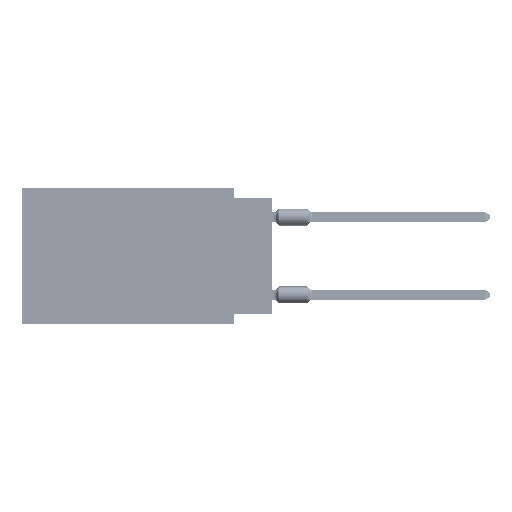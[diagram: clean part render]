
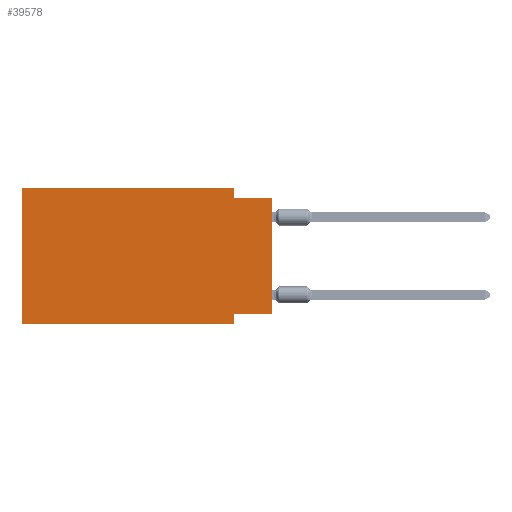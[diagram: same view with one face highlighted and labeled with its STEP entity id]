
A CAD part, left-side view. The second image highlights one B-rep face of the part: STEP entity #39578.
In plain terms, the highlighted planar face has unit normal (-1, 0, 0).
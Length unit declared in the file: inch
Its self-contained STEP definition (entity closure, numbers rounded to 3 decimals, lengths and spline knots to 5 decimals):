
#1362 = VERTEX_POINT ( 'NONE', #86195 ) ;
#1714 = DIRECTION ( 'NONE',  ( 0., -1., 0. ) ) ;
#3912 = EDGE_CURVE ( 'NONE', #1362, #72375, #49674, .T. ) ;
#4605 = CARTESIAN_POINT ( 'NONE',  ( 0., 0.1, 0. ) ) ;
#5267 = CARTESIAN_POINT ( 'NONE',  ( 0., 0., -0.025 ) ) ;
#7550 = CARTESIAN_POINT ( 'NONE',  ( 0., 0.645, 0. ) ) ;
#8729 = CARTESIAN_POINT ( 'NONE',  ( 0., 0.645, 0. ) ) ;
#9142 = LINE ( 'NONE', #7550, #26020 ) ;
#12862 = CARTESIAN_POINT ( 'NONE',  ( 0., 0.645, 0. ) ) ;
#16244 = DIRECTION ( 'NONE',  ( 0., 0., 1. ) ) ;
#19737 = CARTESIAN_POINT ( 'NONE',  ( 0., 0.1, -0.35 ) ) ;
#21460 = EDGE_CURVE ( 'NONE', #58977, #82890, #29327, .T. ) ;
#22205 = VERTEX_POINT ( 'NONE', #104727 ) ;
#22870 = LINE ( 'NONE', #71292, #58501 ) ;
#23210 = ORIENTED_EDGE ( 'NONE', *, *, #62067, .T. ) ;
#23271 = VERTEX_POINT ( 'NONE', #83440 ) ;
#23874 = CARTESIAN_POINT ( 'NONE',  ( 0., 0.1, -0.025 ) ) ;
#24362 = CARTESIAN_POINT ( 'NONE',  ( 0., 0.645, 0. ) ) ;
#26020 = VECTOR ( 'NONE', #67216, 39.37008 ) ;
#29327 = LINE ( 'NONE', #4605, #31275 ) ;
#29997 = VERTEX_POINT ( 'NONE', #53383 ) ;
#31275 = VECTOR ( 'NONE', #70201, 39.37008 ) ;
#31969 = VERTEX_POINT ( 'NONE', #24362 ) ;
#35643 = CARTESIAN_POINT ( 'NONE',  ( 0., 0.1, -0.35 ) ) ;
#38148 = DIRECTION ( 'NONE',  ( 0., 0., -1. ) ) ;
#39578 = ADVANCED_FACE ( 'NONE', ( #69886 ), #61796, .F. ) ;
#42580 = LINE ( 'NONE', #5267, #50592 ) ;
#45679 = DIRECTION ( 'NONE',  ( 1., 0., 0. ) ) ;
#49674 = LINE ( 'NONE', #35643, #68982 ) ;
#50445 = VECTOR ( 'NONE', #51310, 39.37008 ) ;
#50592 = VECTOR ( 'NONE', #1714, 39.37008 ) ;
#51310 = DIRECTION ( 'NONE',  ( 0., -1., 0. ) ) ;
#53383 = CARTESIAN_POINT ( 'NONE',  ( 0., 0., -0.325 ) ) ;
#57918 = CARTESIAN_POINT ( 'NONE',  ( 0., 0., -0.325 ) ) ;
#58501 = VECTOR ( 'NONE', #64800, 39.37008 ) ;
#58977 = VERTEX_POINT ( 'NONE', #88517 ) ;
#59296 = DIRECTION ( 'NONE',  ( 0., 0., -1. ) ) ;
#61796 = PLANE ( 'NONE',  #67469 ) ;
#62067 = EDGE_CURVE ( 'NONE', #23271, #72375, #84107, .T. ) ;
#64331 = EDGE_CURVE ( 'NONE', #82890, #22205, #42580, .T. ) ;
#64800 = DIRECTION ( 'NONE',  ( 0., 0., 1. ) ) ;
#66525 = DIRECTION ( 'NONE',  ( 0., 1., 0. ) ) ;
#66859 = VECTOR ( 'NONE', #16244, 39.37008 ) ;
#67216 = DIRECTION ( 'NONE',  ( 0., -1., 0. ) ) ;
#67469 = AXIS2_PLACEMENT_3D ( 'NONE', #12862, #45679, #38148 ) ;
#68235 = ORIENTED_EDGE ( 'NONE', *, *, #104474, .F. ) ;
#68982 = VECTOR ( 'NONE', #59296, 39.37008 ) ;
#69886 = FACE_OUTER_BOUND ( 'NONE', #101928, .T. ) ;
#70201 = DIRECTION ( 'NONE',  ( 0., 0., -1. ) ) ;
#70419 = VECTOR ( 'NONE', #66525, 39.37008 ) ;
#70621 = ORIENTED_EDGE ( 'NONE', *, *, #21460, .F. ) ;
#71292 = CARTESIAN_POINT ( 'NONE',  ( 0., 0., 0. ) ) ;
#72375 = VERTEX_POINT ( 'NONE', #19737 ) ;
#73145 = ORIENTED_EDGE ( 'NONE', *, *, #105015, .F. ) ;
#74070 = LINE ( 'NONE', #57918, #70419 ) ;
#74323 = LINE ( 'NONE', #8729, #66859 ) ;
#77754 = ORIENTED_EDGE ( 'NONE', *, *, #105225, .T. ) ;
#78158 = CARTESIAN_POINT ( 'NONE',  ( 0., 0.645, -0.35 ) ) ;
#82890 = VERTEX_POINT ( 'NONE', #23874 ) ;
#83440 = CARTESIAN_POINT ( 'NONE',  ( 0., 0.645, -0.35 ) ) ;
#84107 = LINE ( 'NONE', #78158, #50445 ) ;
#86195 = CARTESIAN_POINT ( 'NONE',  ( 0., 0.1, -0.325 ) ) ;
#88517 = CARTESIAN_POINT ( 'NONE',  ( 0., 0.1, 0. ) ) ;
#90219 = ORIENTED_EDGE ( 'NONE', *, *, #64331, .F. ) ;
#97885 = ORIENTED_EDGE ( 'NONE', *, *, #3912, .F. ) ;
#101928 = EDGE_LOOP ( 'NONE', ( #77754, #90219, #70621, #105141, #68235, #23210, #97885, #73145 ) ) ;
#104474 = EDGE_CURVE ( 'NONE', #23271, #31969, #74323, .T. ) ;
#104727 = CARTESIAN_POINT ( 'NONE',  ( 0., 0., -0.025 ) ) ;
#105015 = EDGE_CURVE ( 'NONE', #29997, #1362, #74070, .T. ) ;
#105141 = ORIENTED_EDGE ( 'NONE', *, *, #106136, .F. ) ;
#105225 = EDGE_CURVE ( 'NONE', #29997, #22205, #22870, .T. ) ;
#106136 = EDGE_CURVE ( 'NONE', #31969, #58977, #9142, .T. ) ;
